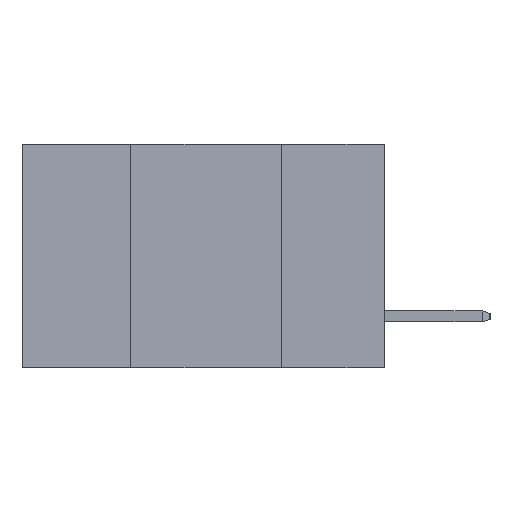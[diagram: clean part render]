
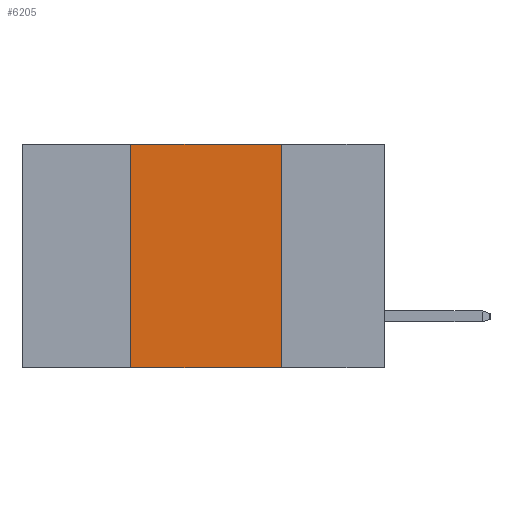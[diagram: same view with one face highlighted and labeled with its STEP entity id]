
A CAD part, left-side view. The second image highlights one B-rep face of the part: STEP entity #6205.
In plain terms, the highlighted planar face has unit normal (-1, 0, 0).
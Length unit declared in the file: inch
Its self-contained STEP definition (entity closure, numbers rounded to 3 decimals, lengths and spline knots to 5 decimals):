
#215 = CARTESIAN_POINT ( 'NONE',  ( 0., 0.42, 0. ) ) ;
#309 = CARTESIAN_POINT ( 'NONE',  ( 0., 0.6, -0.37 ) ) ;
#642 = CARTESIAN_POINT ( 'NONE',  ( 0., 0.17, 0. ) ) ;
#1641 = EDGE_CURVE ( 'NONE', #6393, #16665, #2135, .T. ) ;
#2135 = LINE ( 'NONE', #309, #15910 ) ;
#2143 = PLANE ( 'NONE',  #12766 ) ;
#2158 = VECTOR ( 'NONE', #3844, 39.37008 ) ;
#2445 = EDGE_LOOP ( 'NONE', ( #2877, #3325, #7387, #8250 ) ) ;
#2627 = VECTOR ( 'NONE', #14875, 39.37008 ) ;
#2877 = ORIENTED_EDGE ( 'NONE', *, *, #9041, .F. ) ;
#3325 = ORIENTED_EDGE ( 'NONE', *, *, #8711, .F. ) ;
#3844 = DIRECTION ( 'NONE',  ( 0., -1., 0. ) ) ;
#3909 = VECTOR ( 'NONE', #13877, 39.37008 ) ;
#4194 = CARTESIAN_POINT ( 'NONE',  ( 0., 0.42, -0.37 ) ) ;
#4557 = CARTESIAN_POINT ( 'NONE',  ( 0., 0.17, 0. ) ) ;
#6205 = ADVANCED_FACE ( 'NONE', ( #9888 ), #2143, .F. ) ;
#6393 = VERTEX_POINT ( 'NONE', #4194 ) ;
#7334 = VERTEX_POINT ( 'NONE', #642 ) ;
#7387 = ORIENTED_EDGE ( 'NONE', *, *, #8254, .F. ) ;
#7674 = CARTESIAN_POINT ( 'NONE',  ( 0., 0.6, 0. ) ) ;
#7735 = DIRECTION ( 'NONE',  ( 0., 0., -1. ) ) ;
#7767 = DIRECTION ( 'NONE',  ( 1., 0., 0. ) ) ;
#7813 = VERTEX_POINT ( 'NONE', #215 ) ;
#8250 = ORIENTED_EDGE ( 'NONE', *, *, #1641, .T. ) ;
#8254 = EDGE_CURVE ( 'NONE', #6393, #7813, #9908, .T. ) ;
#8711 = EDGE_CURVE ( 'NONE', #7813, #7334, #16326, .T. ) ;
#9041 = EDGE_CURVE ( 'NONE', #7334, #16665, #11517, .T. ) ;
#9888 = FACE_OUTER_BOUND ( 'NONE', #2445, .T. ) ;
#9908 = LINE ( 'NONE', #16171, #2627 ) ;
#11517 = LINE ( 'NONE', #4557, #3909 ) ;
#12766 = AXIS2_PLACEMENT_3D ( 'NONE', #7674, #7767, #7735 ) ;
#13217 = CARTESIAN_POINT ( 'NONE',  ( 0., 0.6, 0. ) ) ;
#13877 = DIRECTION ( 'NONE',  ( 0., 0., -1. ) ) ;
#14064 = DIRECTION ( 'NONE',  ( 0., -1., 0. ) ) ;
#14875 = DIRECTION ( 'NONE',  ( 0., 0., 1. ) ) ;
#15247 = CARTESIAN_POINT ( 'NONE',  ( 0., 0.17, -0.37 ) ) ;
#15910 = VECTOR ( 'NONE', #14064, 39.37008 ) ;
#16171 = CARTESIAN_POINT ( 'NONE',  ( 0., 0.42, 0. ) ) ;
#16326 = LINE ( 'NONE', #13217, #2158 ) ;
#16665 = VERTEX_POINT ( 'NONE', #15247 ) ;
